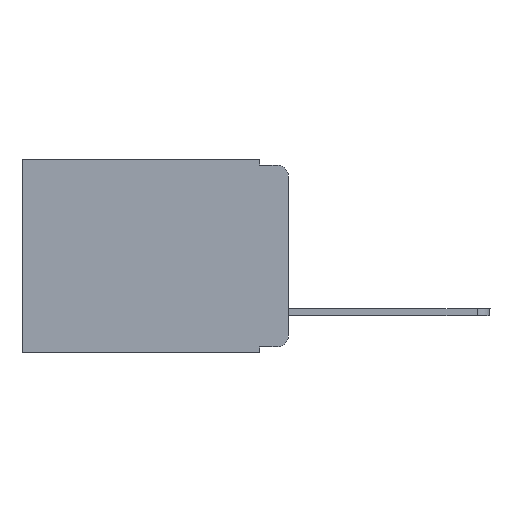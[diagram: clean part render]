
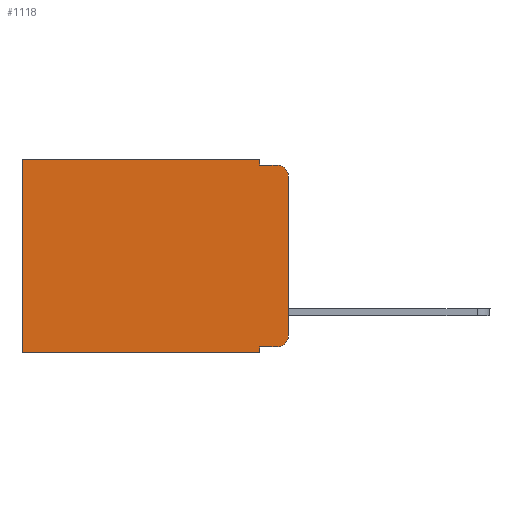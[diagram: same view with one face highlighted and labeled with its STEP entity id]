
A CAD part, left-side view. The second image highlights one B-rep face of the part: STEP entity #1118.
In plain terms, the highlighted planar face has unit normal (-1, 0, 0).
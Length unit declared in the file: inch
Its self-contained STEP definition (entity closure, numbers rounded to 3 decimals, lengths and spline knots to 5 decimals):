
#8 = VERTEX_POINT ( 'NONE', #12008 ) ;
#141 = EDGE_CURVE ( 'NONE', #6858, #9647, #11891, .T. ) ;
#177 = AXIS2_PLACEMENT_3D ( 'NONE', #2798, #1728, #11291 ) ;
#440 = VECTOR ( 'NONE', #9002, 39.37008 ) ;
#581 = EDGE_CURVE ( 'NONE', #8538, #1632, #9729, .T. ) ;
#635 = VECTOR ( 'NONE', #10785, 39.37008 ) ;
#871 = ORIENTED_EDGE ( 'NONE', *, *, #5990, .F. ) ;
#1021 = ORIENTED_EDGE ( 'NONE', *, *, #11861, .T. ) ;
#1118 = ADVANCED_FACE ( 'NONE', ( #2939 ), #1694, .F. ) ;
#1632 = VERTEX_POINT ( 'NONE', #10057 ) ;
#1694 = PLANE ( 'NONE',  #6244 ) ;
#1728 = DIRECTION ( 'NONE',  ( -1., 0., 0. ) ) ;
#1738 = EDGE_CURVE ( 'NONE', #7621, #10471, #7718, .T. ) ;
#2165 = LINE ( 'NONE', #12810, #11082 ) ;
#2314 = VECTOR ( 'NONE', #8185, 39.37008 ) ;
#2498 = LINE ( 'NONE', #8234, #2314 ) ;
#2767 = DIRECTION ( 'NONE',  ( 1., 0., 0. ) ) ;
#2790 = VECTOR ( 'NONE', #11958, 39.37008 ) ;
#2798 = CARTESIAN_POINT ( 'NONE',  ( 0.298, 0.02, -0.313 ) ) ;
#2939 = FACE_OUTER_BOUND ( 'NONE', #5767, .T. ) ;
#3393 = VECTOR ( 'NONE', #7025, 39.37008 ) ;
#3883 = DIRECTION ( 'NONE',  ( 0., 0., -1. ) ) ;
#4750 = LINE ( 'NONE', #7966, #3393 ) ;
#4907 = VERTEX_POINT ( 'NONE', #10164 ) ;
#5095 = CARTESIAN_POINT ( 'NONE',  ( 0.298, 0., -0.03 ) ) ;
#5414 = CIRCLE ( 'NONE', #7409, 0.02 ) ;
#5615 = CARTESIAN_POINT ( 'NONE',  ( 0.298, 0.051, -0.343 ) ) ;
#5730 = DIRECTION ( 'NONE',  ( 0., 0., -1. ) ) ;
#5767 = EDGE_LOOP ( 'NONE', ( #7757, #1021, #11919, #13410, #10607, #6521, #871, #12124, #10594, #9451 ) ) ;
#5783 = CARTESIAN_POINT ( 'NONE',  ( 0.298, 0.051, -0.333 ) ) ;
#5990 = EDGE_CURVE ( 'NONE', #6753, #8, #8348, .T. ) ;
#6037 = VERTEX_POINT ( 'NONE', #12097 ) ;
#6244 = AXIS2_PLACEMENT_3D ( 'NONE', #9086, #2767, #5730 ) ;
#6460 = DIRECTION ( 'NONE',  ( 0., 0., -1. ) ) ;
#6521 = ORIENTED_EDGE ( 'NONE', *, *, #12177, .T. ) ;
#6753 = VERTEX_POINT ( 'NONE', #5615 ) ;
#6858 = VERTEX_POINT ( 'NONE', #13097 ) ;
#7025 = DIRECTION ( 'NONE',  ( 0., 1., 0. ) ) ;
#7084 = DIRECTION ( 'NONE',  ( -1., 0., 0. ) ) ;
#7133 = CARTESIAN_POINT ( 'NONE',  ( 0.298, 0.02, -0.03 ) ) ;
#7409 = AXIS2_PLACEMENT_3D ( 'NONE', #7133, #7084, #3883 ) ;
#7621 = VERTEX_POINT ( 'NONE', #5095 ) ;
#7718 = LINE ( 'NONE', #9461, #9721 ) ;
#7757 = ORIENTED_EDGE ( 'NONE', *, *, #1738, .F. ) ;
#7966 = CARTESIAN_POINT ( 'NONE',  ( 0.298, 0., 0. ) ) ;
#8067 = DIRECTION ( 'NONE',  ( 0., 0., -1. ) ) ;
#8185 = DIRECTION ( 'NONE',  ( 0., -1., 0. ) ) ;
#8234 = CARTESIAN_POINT ( 'NONE',  ( 0.298, 0.051, -0.01 ) ) ;
#8261 = DIRECTION ( 'NONE',  ( 0., 0., -1. ) ) ;
#8348 = LINE ( 'NONE', #9911, #440 ) ;
#8538 = VERTEX_POINT ( 'NONE', #5783 ) ;
#8753 = CARTESIAN_POINT ( 'NONE',  ( 0.298, 0.051, -0.333 ) ) ;
#8952 = CARTESIAN_POINT ( 'NONE',  ( 0.298, 0.051, 0. ) ) ;
#9002 = DIRECTION ( 'NONE',  ( 0., 1., 0. ) ) ;
#9086 = CARTESIAN_POINT ( 'NONE',  ( 0.298, 0., 0. ) ) ;
#9319 = EDGE_CURVE ( 'NONE', #9647, #6037, #2498, .T. ) ;
#9414 = EDGE_CURVE ( 'NONE', #8538, #6753, #2165, .T. ) ;
#9451 = ORIENTED_EDGE ( 'NONE', *, *, #10699, .T. ) ;
#9461 = CARTESIAN_POINT ( 'NONE',  ( 0.298, 0., 0. ) ) ;
#9582 = CARTESIAN_POINT ( 'NONE',  ( 0.298, 0.473, 0. ) ) ;
#9647 = VERTEX_POINT ( 'NONE', #10156 ) ;
#9721 = VECTOR ( 'NONE', #8261, 39.37008 ) ;
#9729 = LINE ( 'NONE', #8753, #2790 ) ;
#9801 = CARTESIAN_POINT ( 'NONE',  ( 0.298, 0., -0.313 ) ) ;
#9911 = CARTESIAN_POINT ( 'NONE',  ( 0.298, 0., -0.343 ) ) ;
#10057 = CARTESIAN_POINT ( 'NONE',  ( 0.298, 0.02, -0.333 ) ) ;
#10156 = CARTESIAN_POINT ( 'NONE',  ( 0.298, 0.051, -0.01 ) ) ;
#10164 = CARTESIAN_POINT ( 'NONE',  ( 0.298, 0.473, 0. ) ) ;
#10471 = VERTEX_POINT ( 'NONE', #9801 ) ;
#10594 = ORIENTED_EDGE ( 'NONE', *, *, #581, .T. ) ;
#10607 = ORIENTED_EDGE ( 'NONE', *, *, #12475, .T. ) ;
#10699 = EDGE_CURVE ( 'NONE', #1632, #10471, #11047, .T. ) ;
#10785 = DIRECTION ( 'NONE',  ( 0., 0., -1. ) ) ;
#10883 = VECTOR ( 'NONE', #8067, 39.37008 ) ;
#11047 = CIRCLE ( 'NONE', #177, 0.02 ) ;
#11082 = VECTOR ( 'NONE', #6460, 39.37008 ) ;
#11291 = DIRECTION ( 'NONE',  ( 0., 0., -1. ) ) ;
#11861 = EDGE_CURVE ( 'NONE', #7621, #6037, #5414, .T. ) ;
#11891 = LINE ( 'NONE', #8952, #10883 ) ;
#11919 = ORIENTED_EDGE ( 'NONE', *, *, #9319, .F. ) ;
#11958 = DIRECTION ( 'NONE',  ( 0., -1., 0. ) ) ;
#12008 = CARTESIAN_POINT ( 'NONE',  ( 0.298, 0.473, -0.343 ) ) ;
#12097 = CARTESIAN_POINT ( 'NONE',  ( 0.298, 0.02, -0.01 ) ) ;
#12124 = ORIENTED_EDGE ( 'NONE', *, *, #9414, .F. ) ;
#12177 = EDGE_CURVE ( 'NONE', #4907, #8, #12999, .T. ) ;
#12475 = EDGE_CURVE ( 'NONE', #6858, #4907, #4750, .T. ) ;
#12810 = CARTESIAN_POINT ( 'NONE',  ( 0.298, 0.051, 0. ) ) ;
#12999 = LINE ( 'NONE', #9582, #635 ) ;
#13097 = CARTESIAN_POINT ( 'NONE',  ( 0.298, 0.051, 0. ) ) ;
#13410 = ORIENTED_EDGE ( 'NONE', *, *, #141, .F. ) ;
